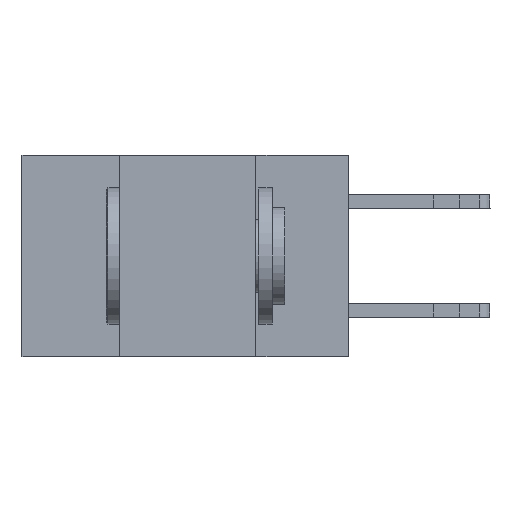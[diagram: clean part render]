
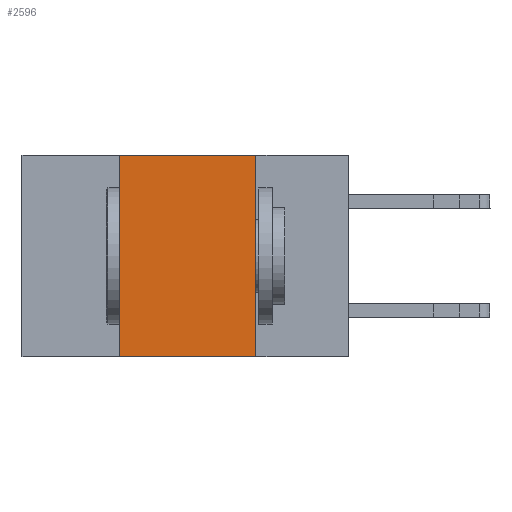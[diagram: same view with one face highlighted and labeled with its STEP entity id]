
A CAD part, left-side view. The second image highlights one B-rep face of the part: STEP entity #2596.
In plain terms, the highlighted planar face has unit normal (-1, 0, 0).
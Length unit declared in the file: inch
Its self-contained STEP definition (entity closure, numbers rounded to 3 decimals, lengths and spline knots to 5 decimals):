
#428 = CARTESIAN_POINT ( 'NONE',  ( 0., 0.42, -0.37 ) ) ;
#749 = CARTESIAN_POINT ( 'NONE',  ( 0., 0.6, 0. ) ) ;
#868 = VERTEX_POINT ( 'NONE', #12497 ) ;
#1212 = DIRECTION ( 'NONE',  ( 1., 0., 0. ) ) ;
#1425 = VERTEX_POINT ( 'NONE', #5230 ) ;
#1973 = FACE_OUTER_BOUND ( 'NONE', #4280, .T. ) ;
#2008 = DIRECTION ( 'NONE',  ( 0., 0., -1. ) ) ;
#2293 = ORIENTED_EDGE ( 'NONE', *, *, #10953, .F. ) ;
#2462 = EDGE_CURVE ( 'NONE', #868, #1425, #12211, .T. ) ;
#2596 = ADVANCED_FACE ( 'NONE', ( #1973 ), #12339, .F. ) ;
#2862 = CARTESIAN_POINT ( 'NONE',  ( 0., 0.17, -0.37 ) ) ;
#4280 = EDGE_LOOP ( 'NONE', ( #10216, #11885, #2293, #10502 ) ) ;
#4476 = DIRECTION ( 'NONE',  ( 0., -1., 0. ) ) ;
#4720 = VERTEX_POINT ( 'NONE', #2862 ) ;
#5108 = EDGE_CURVE ( 'NONE', #9816, #4720, #7022, .T. ) ;
#5189 = DIRECTION ( 'NONE',  ( 0., 0., 1. ) ) ;
#5230 = CARTESIAN_POINT ( 'NONE',  ( 0., 0.17, 0. ) ) ;
#5370 = VECTOR ( 'NONE', #5189, 39.37008 ) ;
#5824 = VECTOR ( 'NONE', #2008, 39.37008 ) ;
#5874 = VECTOR ( 'NONE', #4476, 39.37008 ) ;
#7022 = LINE ( 'NONE', #12200, #5874 ) ;
#8345 = LINE ( 'NONE', #12438, #5370 ) ;
#9316 = CARTESIAN_POINT ( 'NONE',  ( 0., 0.6, 0. ) ) ;
#9816 = VERTEX_POINT ( 'NONE', #428 ) ;
#10216 = ORIENTED_EDGE ( 'NONE', *, *, #12486, .F. ) ;
#10502 = ORIENTED_EDGE ( 'NONE', *, *, #5108, .T. ) ;
#10953 = EDGE_CURVE ( 'NONE', #9816, #868, #8345, .T. ) ;
#11173 = CARTESIAN_POINT ( 'NONE',  ( 0., 0.17, 0. ) ) ;
#11262 = DIRECTION ( 'NONE',  ( 0., 0., -1. ) ) ;
#11885 = ORIENTED_EDGE ( 'NONE', *, *, #2462, .F. ) ;
#12011 = DIRECTION ( 'NONE',  ( 0., -1., 0. ) ) ;
#12176 = LINE ( 'NONE', #11173, #5824 ) ;
#12200 = CARTESIAN_POINT ( 'NONE',  ( 0., 0.6, -0.37 ) ) ;
#12211 = LINE ( 'NONE', #749, #13166 ) ;
#12339 = PLANE ( 'NONE',  #12512 ) ;
#12438 = CARTESIAN_POINT ( 'NONE',  ( 0., 0.42, 0. ) ) ;
#12486 = EDGE_CURVE ( 'NONE', #1425, #4720, #12176, .T. ) ;
#12497 = CARTESIAN_POINT ( 'NONE',  ( 0., 0.42, 0. ) ) ;
#12512 = AXIS2_PLACEMENT_3D ( 'NONE', #9316, #1212, #11262 ) ;
#13166 = VECTOR ( 'NONE', #12011, 39.37008 ) ;
